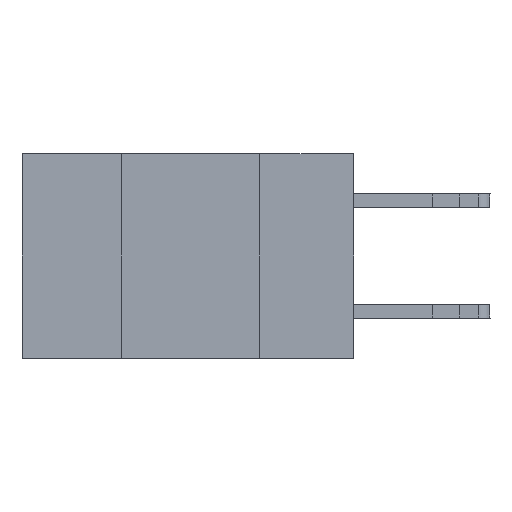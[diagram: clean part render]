
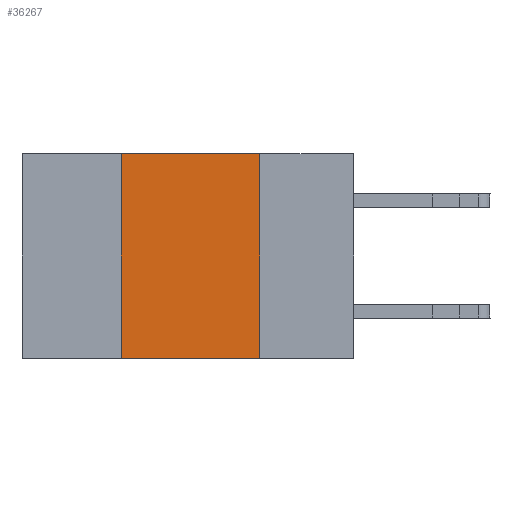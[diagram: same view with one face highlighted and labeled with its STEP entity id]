
A CAD part, left-side view. The second image highlights one B-rep face of the part: STEP entity #36267.
In plain terms, the highlighted planar face has unit normal (-1, 0, 0).
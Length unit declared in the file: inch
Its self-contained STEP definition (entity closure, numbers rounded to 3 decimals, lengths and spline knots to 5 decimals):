
#50 = AXIS2_PLACEMENT_3D ( 'NONE', #3900, #28434, #38157 ) ;
#2562 = DIRECTION ( 'NONE',  ( 0., -1., 0. ) ) ;
#3900 = CARTESIAN_POINT ( 'NONE',  ( 0., 0.6, 0. ) ) ;
#4157 = VECTOR ( 'NONE', #27710, 39.37008 ) ;
#4843 = CARTESIAN_POINT ( 'NONE',  ( 0., 0.6, 0. ) ) ;
#8771 = VECTOR ( 'NONE', #29903, 39.37008 ) ;
#9936 = EDGE_CURVE ( 'NONE', #11793, #38489, #38666, .T. ) ;
#11722 = CARTESIAN_POINT ( 'NONE',  ( 0., 0.6, -0.37 ) ) ;
#11793 = VERTEX_POINT ( 'NONE', #33252 ) ;
#12607 = ORIENTED_EDGE ( 'NONE', *, *, #32591, .F. ) ;
#13073 = VERTEX_POINT ( 'NONE', #24338 ) ;
#14797 = CARTESIAN_POINT ( 'NONE',  ( 0., 0.17, 0. ) ) ;
#15992 = EDGE_CURVE ( 'NONE', #13073, #38489, #24049, .T. ) ;
#17075 = VECTOR ( 'NONE', #24094, 39.37008 ) ;
#17404 = CARTESIAN_POINT ( 'NONE',  ( 0., 0.17, -0.37 ) ) ;
#17463 = LINE ( 'NONE', #4843, #8771 ) ;
#18314 = EDGE_CURVE ( 'NONE', #19878, #13073, #17463, .T. ) ;
#19878 = VERTEX_POINT ( 'NONE', #28431 ) ;
#23430 = LINE ( 'NONE', #36239, #17075 ) ;
#24049 = LINE ( 'NONE', #14797, #4157 ) ;
#24094 = DIRECTION ( 'NONE',  ( 0., 0., 1. ) ) ;
#24175 = VECTOR ( 'NONE', #2562, 39.37008 ) ;
#24338 = CARTESIAN_POINT ( 'NONE',  ( 0., 0.17, 0. ) ) ;
#27710 = DIRECTION ( 'NONE',  ( 0., 0., -1. ) ) ;
#28431 = CARTESIAN_POINT ( 'NONE',  ( 0., 0.42, 0. ) ) ;
#28434 = DIRECTION ( 'NONE',  ( 1., 0., 0. ) ) ;
#29695 = ORIENTED_EDGE ( 'NONE', *, *, #15992, .F. ) ;
#29903 = DIRECTION ( 'NONE',  ( 0., -1., 0. ) ) ;
#29956 = FACE_OUTER_BOUND ( 'NONE', #33310, .T. ) ;
#31813 = PLANE ( 'NONE',  #50 ) ;
#32591 = EDGE_CURVE ( 'NONE', #11793, #19878, #23430, .T. ) ;
#33252 = CARTESIAN_POINT ( 'NONE',  ( 0., 0.42, -0.37 ) ) ;
#33310 = EDGE_LOOP ( 'NONE', ( #29695, #39745, #12607, #33988 ) ) ;
#33988 = ORIENTED_EDGE ( 'NONE', *, *, #9936, .T. ) ;
#36239 = CARTESIAN_POINT ( 'NONE',  ( 0., 0.42, 0. ) ) ;
#36267 = ADVANCED_FACE ( 'NONE', ( #29956 ), #31813, .F. ) ;
#38157 = DIRECTION ( 'NONE',  ( 0., 0., -1. ) ) ;
#38489 = VERTEX_POINT ( 'NONE', #17404 ) ;
#38666 = LINE ( 'NONE', #11722, #24175 ) ;
#39745 = ORIENTED_EDGE ( 'NONE', *, *, #18314, .F. ) ;
